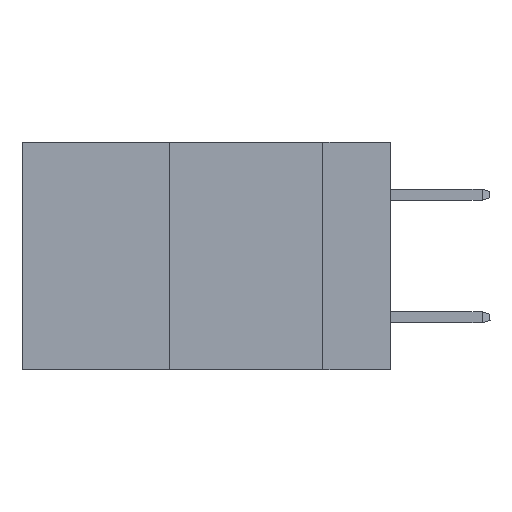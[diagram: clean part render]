
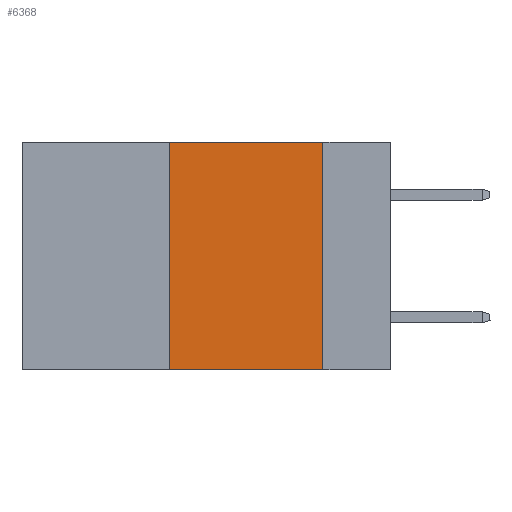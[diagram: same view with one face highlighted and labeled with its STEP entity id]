
A CAD part, left-side view. The second image highlights one B-rep face of the part: STEP entity #6368.
In plain terms, the highlighted planar face has unit normal (-1, 0, 0).
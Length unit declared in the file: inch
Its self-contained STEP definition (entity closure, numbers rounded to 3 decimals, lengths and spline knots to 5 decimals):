
#227 = DIRECTION ( 'NONE',  ( 0., 0., -1. ) ) ;
#1192 = VECTOR ( 'NONE', #4277, 39.37008 ) ;
#1813 = ORIENTED_EDGE ( 'NONE', *, *, #7322, .F. ) ;
#2213 = EDGE_CURVE ( 'NONE', #3404, #4149, #4779, .T. ) ;
#2625 = AXIS2_PLACEMENT_3D ( 'NONE', #9038, #8056, #227 ) ;
#2995 = DIRECTION ( 'NONE',  ( 0., 0., 1. ) ) ;
#3300 = CARTESIAN_POINT ( 'NONE',  ( 0., 0.11, 0. ) ) ;
#3404 = VERTEX_POINT ( 'NONE', #9633 ) ;
#3405 = EDGE_CURVE ( 'NONE', #9928, #9399, #8204, .T. ) ;
#3428 = CARTESIAN_POINT ( 'NONE',  ( 0., 0.11, -0.37 ) ) ;
#4149 = VERTEX_POINT ( 'NONE', #3300 ) ;
#4277 = DIRECTION ( 'NONE',  ( 0., 0., -1. ) ) ;
#4377 = LINE ( 'NONE', #10207, #4499 ) ;
#4443 = ORIENTED_EDGE ( 'NONE', *, *, #6819, .F. ) ;
#4499 = VECTOR ( 'NONE', #2995, 39.37008 ) ;
#4779 = LINE ( 'NONE', #7623, #6919 ) ;
#5507 = LINE ( 'NONE', #9736, #1192 ) ;
#5649 = DIRECTION ( 'NONE',  ( 0., -1., 0. ) ) ;
#5914 = ORIENTED_EDGE ( 'NONE', *, *, #2213, .F. ) ;
#6304 = FACE_OUTER_BOUND ( 'NONE', #7118, .T. ) ;
#6368 = ADVANCED_FACE ( 'NONE', ( #6304 ), #7312, .F. ) ;
#6819 = EDGE_CURVE ( 'NONE', #9928, #3404, #4377, .T. ) ;
#6919 = VECTOR ( 'NONE', #7720, 39.37008 ) ;
#7118 = EDGE_LOOP ( 'NONE', ( #1813, #5914, #4443, #9562 ) ) ;
#7236 = CARTESIAN_POINT ( 'NONE',  ( 0., 0.6, -0.37 ) ) ;
#7312 = PLANE ( 'NONE',  #2625 ) ;
#7322 = EDGE_CURVE ( 'NONE', #4149, #9399, #5507, .T. ) ;
#7623 = CARTESIAN_POINT ( 'NONE',  ( 0., 0.6, 0. ) ) ;
#7720 = DIRECTION ( 'NONE',  ( 0., -1., 0. ) ) ;
#8056 = DIRECTION ( 'NONE',  ( 1., 0., 0. ) ) ;
#8067 = VECTOR ( 'NONE', #5649, 39.37008 ) ;
#8204 = LINE ( 'NONE', #7236, #8067 ) ;
#8653 = CARTESIAN_POINT ( 'NONE',  ( 0., 0.36, -0.37 ) ) ;
#9038 = CARTESIAN_POINT ( 'NONE',  ( 0., 0.6, 0. ) ) ;
#9399 = VERTEX_POINT ( 'NONE', #3428 ) ;
#9562 = ORIENTED_EDGE ( 'NONE', *, *, #3405, .T. ) ;
#9633 = CARTESIAN_POINT ( 'NONE',  ( 0., 0.36, 0. ) ) ;
#9736 = CARTESIAN_POINT ( 'NONE',  ( 0., 0.11, 0. ) ) ;
#9928 = VERTEX_POINT ( 'NONE', #8653 ) ;
#10207 = CARTESIAN_POINT ( 'NONE',  ( 0., 0.36, 0. ) ) ;
